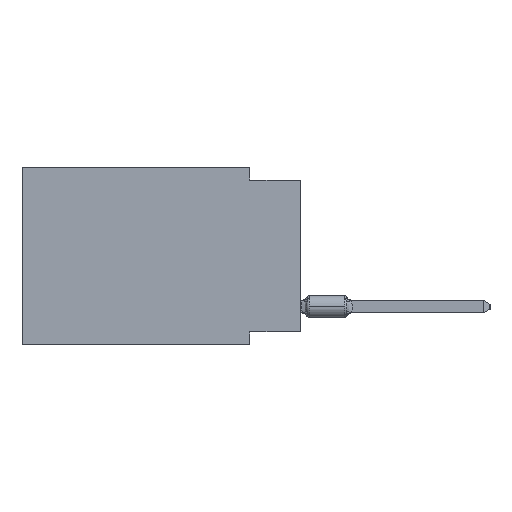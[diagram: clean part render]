
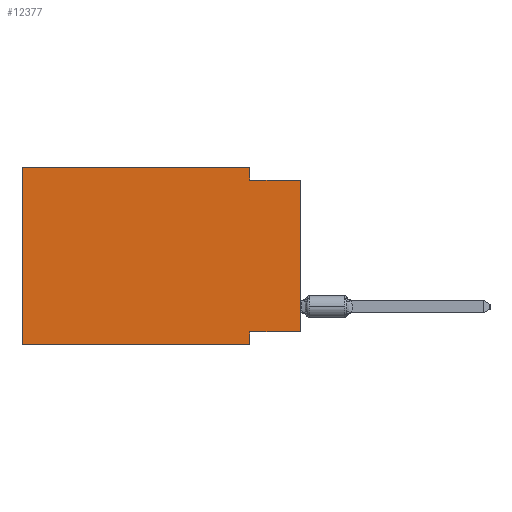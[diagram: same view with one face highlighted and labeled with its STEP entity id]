
A CAD part, left-side view. The second image highlights one B-rep face of the part: STEP entity #12377.
In plain terms, the highlighted planar face has unit normal (-1, 0, 0).
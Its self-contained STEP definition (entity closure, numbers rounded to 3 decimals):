
#47 = LINE ( 'NONE', #10065, #20149 ) ;
#154 = FACE_OUTER_BOUND ( 'NONE', #6305, .T. ) ;
#165 = ORIENTED_EDGE ( 'NONE', *, *, #21131, .F. ) ;
#175 = EDGE_CURVE ( 'NONE', #25934, #17260, #4139, .T. ) ;
#216 = DIRECTION ( 'NONE',  ( 0., -1., 0. ) ) ;
#1028 = EDGE_CURVE ( 'NONE', #20763, #8382, #24373, .T. ) ;
#2440 = ORIENTED_EDGE ( 'NONE', *, *, #5213, .F. ) ;
#2460 = VERTEX_POINT ( 'NONE', #27641 ) ;
#4139 = LINE ( 'NONE', #11385, #20322 ) ;
#4153 = DIRECTION ( 'NONE',  ( 0., -1., 0. ) ) ;
#4309 = CARTESIAN_POINT ( 'NONE',  ( 0., 13.97, -8.89 ) ) ;
#4961 = CARTESIAN_POINT ( 'NONE',  ( 0., 2.54, 0. ) ) ;
#5029 = DIRECTION ( 'NONE',  ( 0., 0., -1. ) ) ;
#5183 = CARTESIAN_POINT ( 'NONE',  ( 0., 0., -0.635 ) ) ;
#5213 = EDGE_CURVE ( 'NONE', #25964, #25934, #8222, .T. ) ;
#5443 = VECTOR ( 'NONE', #24599, 1000. ) ;
#6130 = DIRECTION ( 'NONE',  ( 0., 1., 0. ) ) ;
#6305 = EDGE_LOOP ( 'NONE', ( #25351, #13534, #31965, #165, #26317, #13546, #23944, #2440 ) ) ;
#6423 = VECTOR ( 'NONE', #4153, 1000. ) ;
#8222 = LINE ( 'NONE', #18412, #31460 ) ;
#8382 = VERTEX_POINT ( 'NONE', #21340 ) ;
#9139 = LINE ( 'NONE', #4309, #6423 ) ;
#9563 = EDGE_CURVE ( 'NONE', #2460, #17260, #9139, .T. ) ;
#9573 = VECTOR ( 'NONE', #216, 1000. ) ;
#9861 = PLANE ( 'NONE',  #14698 ) ;
#10065 = CARTESIAN_POINT ( 'NONE',  ( 0., 13.97, 0. ) ) ;
#11385 = CARTESIAN_POINT ( 'NONE',  ( 0., 2.54, -8.89 ) ) ;
#12291 = VERTEX_POINT ( 'NONE', #18780 ) ;
#12335 = EDGE_CURVE ( 'NONE', #8382, #12291, #12740, .T. ) ;
#12377 = ADVANCED_FACE ( 'NONE', ( #154 ), #9861, .F. ) ;
#12740 = LINE ( 'NONE', #5183, #5443 ) ;
#12904 = DIRECTION ( 'NONE',  ( 1., 0., 0. ) ) ;
#13534 = ORIENTED_EDGE ( 'NONE', *, *, #12335, .F. ) ;
#13546 = ORIENTED_EDGE ( 'NONE', *, *, #9563, .T. ) ;
#14698 = AXIS2_PLACEMENT_3D ( 'NONE', #19893, #12904, #5029 ) ;
#16344 = CARTESIAN_POINT ( 'NONE',  ( 0., 13.97, 0. ) ) ;
#16577 = VERTEX_POINT ( 'NONE', #16344 ) ;
#16915 = DIRECTION ( 'NONE',  ( 0., 0., -1. ) ) ;
#17260 = VERTEX_POINT ( 'NONE', #20161 ) ;
#17361 = CARTESIAN_POINT ( 'NONE',  ( 0., 0., -8.255 ) ) ;
#18412 = CARTESIAN_POINT ( 'NONE',  ( 0., 0., -8.255 ) ) ;
#18780 = CARTESIAN_POINT ( 'NONE',  ( 0., 0., -0.635 ) ) ;
#19893 = CARTESIAN_POINT ( 'NONE',  ( 0., 13.97, 0. ) ) ;
#20149 = VECTOR ( 'NONE', #25260, 1000. ) ;
#20161 = CARTESIAN_POINT ( 'NONE',  ( 0., 2.54, -8.89 ) ) ;
#20322 = VECTOR ( 'NONE', #21266, 1000. ) ;
#20763 = VERTEX_POINT ( 'NONE', #4961 ) ;
#21131 = EDGE_CURVE ( 'NONE', #16577, #20763, #27564, .T. ) ;
#21266 = DIRECTION ( 'NONE',  ( 0., 0., -1. ) ) ;
#21340 = CARTESIAN_POINT ( 'NONE',  ( 0., 2.54, -0.635 ) ) ;
#22220 = CARTESIAN_POINT ( 'NONE',  ( 0., 13.97, 0. ) ) ;
#23944 = ORIENTED_EDGE ( 'NONE', *, *, #175, .F. ) ;
#24373 = LINE ( 'NONE', #31645, #26519 ) ;
#24599 = DIRECTION ( 'NONE',  ( 0., -1., 0. ) ) ;
#24663 = LINE ( 'NONE', #29523, #30471 ) ;
#25126 = CARTESIAN_POINT ( 'NONE',  ( 0., 2.54, -8.255 ) ) ;
#25260 = DIRECTION ( 'NONE',  ( 0., 0., 1. ) ) ;
#25351 = ORIENTED_EDGE ( 'NONE', *, *, #25544, .T. ) ;
#25544 = EDGE_CURVE ( 'NONE', #25964, #12291, #24663, .T. ) ;
#25934 = VERTEX_POINT ( 'NONE', #25126 ) ;
#25964 = VERTEX_POINT ( 'NONE', #17361 ) ;
#26317 = ORIENTED_EDGE ( 'NONE', *, *, #31389, .F. ) ;
#26519 = VECTOR ( 'NONE', #16915, 1000. ) ;
#27564 = LINE ( 'NONE', #22220, #9573 ) ;
#27641 = CARTESIAN_POINT ( 'NONE',  ( 0., 13.97, -8.89 ) ) ;
#29523 = CARTESIAN_POINT ( 'NONE',  ( 0., 0., 0. ) ) ;
#29840 = DIRECTION ( 'NONE',  ( 0., 0., 1. ) ) ;
#30471 = VECTOR ( 'NONE', #29840, 1000. ) ;
#31389 = EDGE_CURVE ( 'NONE', #2460, #16577, #47, .T. ) ;
#31460 = VECTOR ( 'NONE', #6130, 1000. ) ;
#31645 = CARTESIAN_POINT ( 'NONE',  ( 0., 2.54, 0. ) ) ;
#31965 = ORIENTED_EDGE ( 'NONE', *, *, #1028, .F. ) ;
